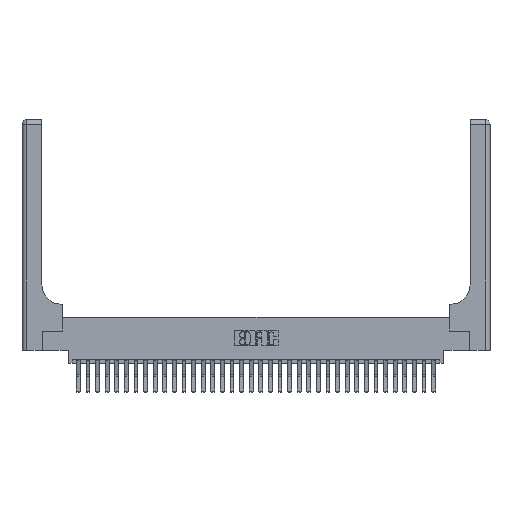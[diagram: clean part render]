
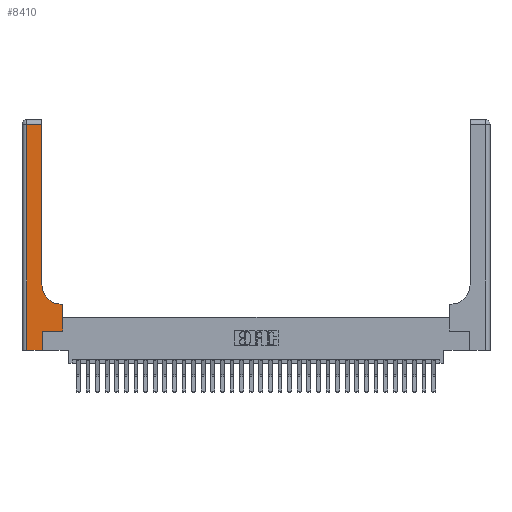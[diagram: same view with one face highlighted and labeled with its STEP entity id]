
A CAD part, top view. The second image highlights one B-rep face of the part: STEP entity #8410.
In plain terms, the highlighted planar face has unit normal (0, 0, 1).
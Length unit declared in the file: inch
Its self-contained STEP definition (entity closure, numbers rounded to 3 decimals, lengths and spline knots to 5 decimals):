
#155 = ORIENTED_EDGE ( 'NONE', *, *, #5830, .T. ) ;
#328 = VERTEX_POINT ( 'NONE', #30388 ) ;
#920 = ORIENTED_EDGE ( 'NONE', *, *, #22505, .T. ) ;
#1022 = FACE_OUTER_BOUND ( 'NONE', #30710, .T. ) ;
#1210 = DIRECTION ( 'NONE',  ( -1., 0., 0. ) ) ;
#2253 = LINE ( 'NONE', #11911, #26051 ) ;
#3546 = VERTEX_POINT ( 'NONE', #5762 ) ;
#3704 = DIRECTION ( 'NONE',  ( 0., 1., 0. ) ) ;
#3872 = VERTEX_POINT ( 'NONE', #12968 ) ;
#3916 = ORIENTED_EDGE ( 'NONE', *, *, #18123, .T. ) ;
#4683 = ORIENTED_EDGE ( 'NONE', *, *, #25466, .T. ) ;
#5126 = EDGE_CURVE ( 'NONE', #29473, #19624, #29133, .T. ) ;
#5762 = CARTESIAN_POINT ( 'NONE',  ( 0.26, 2.94, 0.37 ) ) ;
#5830 = EDGE_CURVE ( 'NONE', #3546, #29473, #28561, .T. ) ;
#6592 = CARTESIAN_POINT ( 'NONE',  ( 0.528, 0.6, 0.37 ) ) ;
#6617 = EDGE_CURVE ( 'NONE', #28082, #29112, #18763, .T. ) ;
#7249 = VECTOR ( 'NONE', #10278, 39.37008 ) ;
#8410 = ADVANCED_FACE ( 'NONE', ( #1022 ), #17789, .F. ) ;
#9010 = AXIS2_PLACEMENT_3D ( 'NONE', #25057, #27415, #15415 ) ;
#9506 = AXIS2_PLACEMENT_3D ( 'NONE', #10830, #20467, #30083 ) ;
#10199 = DIRECTION ( 'NONE',  ( 1., 0., 0. ) ) ;
#10257 = ORIENTED_EDGE ( 'NONE', *, *, #19800, .T. ) ;
#10278 = DIRECTION ( 'NONE',  ( 1., 0., 0. ) ) ;
#10668 = LINE ( 'NONE', #20156, #17269 ) ;
#10830 = CARTESIAN_POINT ( 'NONE',  ( 0.51, 0.85, 0.37 ) ) ;
#11178 = EDGE_CURVE ( 'NONE', #29112, #19311, #22117, .T. ) ;
#11911 = CARTESIAN_POINT ( 'NONE',  ( 0.26, 3., 0.37 ) ) ;
#12086 = DIRECTION ( 'NONE',  ( 0., -1., 0. ) ) ;
#12968 = CARTESIAN_POINT ( 'NONE',  ( 0.528, 0.25, 0.37 ) ) ;
#13389 = CARTESIAN_POINT ( 'NONE',  ( 0.26, 0.6, 0.37 ) ) ;
#14560 = CARTESIAN_POINT ( 'NONE',  ( 0.26, 0.85, 0.37 ) ) ;
#15270 = ORIENTED_EDGE ( 'NONE', *, *, #30117, .T. ) ;
#15415 = DIRECTION ( 'NONE',  ( -1., 0., 0. ) ) ;
#16947 = ORIENTED_EDGE ( 'NONE', *, *, #5126, .T. ) ;
#17269 = VECTOR ( 'NONE', #3704, 39.37008 ) ;
#17685 = LINE ( 'NONE', #29687, #7249 ) ;
#17789 = PLANE ( 'NONE',  #9010 ) ;
#18123 = EDGE_CURVE ( 'NONE', #3872, #28082, #10668, .T. ) ;
#18630 = DIRECTION ( 'NONE',  ( -1., 0., 0. ) ) ;
#18702 = CARTESIAN_POINT ( 'NONE',  ( 0.265, 0., 0.37 ) ) ;
#18763 = LINE ( 'NONE', #13389, #28957 ) ;
#19311 = VERTEX_POINT ( 'NONE', #14560 ) ;
#19578 = ORIENTED_EDGE ( 'NONE', *, *, #11178, .T. ) ;
#19624 = VERTEX_POINT ( 'NONE', #23269 ) ;
#19800 = EDGE_CURVE ( 'NONE', #19624, #25559, #17685, .T. ) ;
#20156 = CARTESIAN_POINT ( 'NONE',  ( 0.528, 0.25, 0.37 ) ) ;
#20467 = DIRECTION ( 'NONE',  ( 0., 0., -1. ) ) ;
#20501 = ORIENTED_EDGE ( 'NONE', *, *, #6617, .T. ) ;
#21559 = VECTOR ( 'NONE', #12086, 39.37008 ) ;
#22117 = CIRCLE ( 'NONE', #9506, 0.25 ) ;
#22358 = LINE ( 'NONE', #29759, #23291 ) ;
#22505 = EDGE_CURVE ( 'NONE', #19311, #3546, #2253, .T. ) ;
#23269 = CARTESIAN_POINT ( 'NONE',  ( 0.06, 0., 0.37 ) ) ;
#23291 = VECTOR ( 'NONE', #10199, 39.37008 ) ;
#23692 = CARTESIAN_POINT ( 'NONE',  ( 0., 2.94, 0.37 ) ) ;
#24966 = DIRECTION ( 'NONE',  ( 0., 1., 0. ) ) ;
#25057 = CARTESIAN_POINT ( 'NONE',  ( 0., 3., 0.37 ) ) ;
#25466 = EDGE_CURVE ( 'NONE', #328, #3872, #22358, .T. ) ;
#25507 = CARTESIAN_POINT ( 'NONE',  ( 0.265, 0., 0.37 ) ) ;
#25559 = VERTEX_POINT ( 'NONE', #25507 ) ;
#26051 = VECTOR ( 'NONE', #24966, 39.37008 ) ;
#26234 = VECTOR ( 'NONE', #18630, 39.37008 ) ;
#26455 = CARTESIAN_POINT ( 'NONE',  ( 0.06, 3., 0.37 ) ) ;
#26690 = CARTESIAN_POINT ( 'NONE',  ( 0.51, 0.6, 0.37 ) ) ;
#27415 = DIRECTION ( 'NONE',  ( 0., 0., -1. ) ) ;
#27864 = DIRECTION ( 'NONE',  ( 0., 1., 0. ) ) ;
#28021 = LINE ( 'NONE', #18702, #28499 ) ;
#28082 = VERTEX_POINT ( 'NONE', #6592 ) ;
#28499 = VECTOR ( 'NONE', #27864, 39.37008 ) ;
#28561 = LINE ( 'NONE', #23692, #26234 ) ;
#28957 = VECTOR ( 'NONE', #1210, 39.37008 ) ;
#29021 = CARTESIAN_POINT ( 'NONE',  ( 0.06, 2.94, 0.37 ) ) ;
#29112 = VERTEX_POINT ( 'NONE', #26690 ) ;
#29133 = LINE ( 'NONE', #26455, #21559 ) ;
#29473 = VERTEX_POINT ( 'NONE', #29021 ) ;
#29687 = CARTESIAN_POINT ( 'NONE',  ( 0., 0., 0.37 ) ) ;
#29759 = CARTESIAN_POINT ( 'NONE',  ( 0.265, 0.25, 0.37 ) ) ;
#30083 = DIRECTION ( 'NONE',  ( 1., 0., 0. ) ) ;
#30117 = EDGE_CURVE ( 'NONE', #25559, #328, #28021, .T. ) ;
#30388 = CARTESIAN_POINT ( 'NONE',  ( 0.265, 0.25, 0.37 ) ) ;
#30710 = EDGE_LOOP ( 'NONE', ( #920, #155, #16947, #10257, #15270, #4683, #3916, #20501, #19578 ) ) ;
